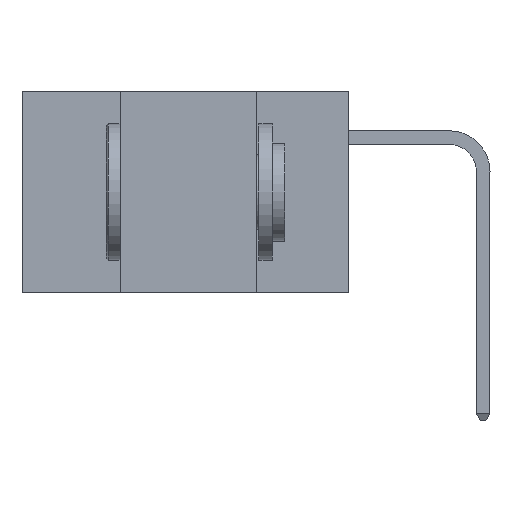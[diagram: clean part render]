
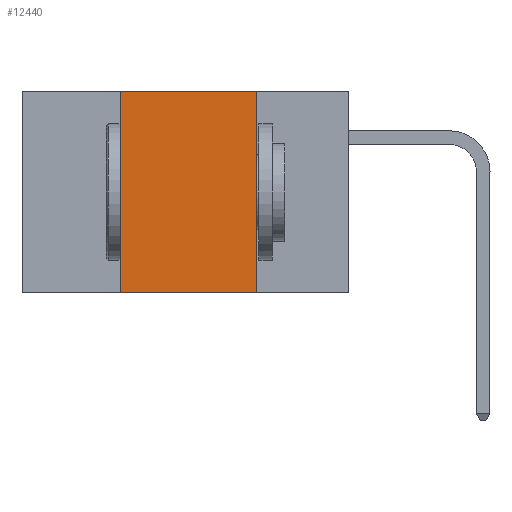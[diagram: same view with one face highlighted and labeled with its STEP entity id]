
A CAD part, left-side view. The second image highlights one B-rep face of the part: STEP entity #12440.
In plain terms, the highlighted planar face has unit normal (-1, 0, 0).
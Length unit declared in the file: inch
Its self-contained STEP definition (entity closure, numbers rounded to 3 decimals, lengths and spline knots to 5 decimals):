
#71 = CARTESIAN_POINT ( 'NONE',  ( 0., 0.6, 0. ) ) ;
#169 = DIRECTION ( 'NONE',  ( 1., 0., 0. ) ) ;
#422 = VECTOR ( 'NONE', #1328, 39.37008 ) ;
#915 = VERTEX_POINT ( 'NONE', #7883 ) ;
#1328 = DIRECTION ( 'NONE',  ( 0., 0., -1. ) ) ;
#1409 = CARTESIAN_POINT ( 'NONE',  ( 0., 0.17, 0. ) ) ;
#1415 = DIRECTION ( 'NONE',  ( 0., 0., 1. ) ) ;
#1425 = CARTESIAN_POINT ( 'NONE',  ( 0., 0.17, 0. ) ) ;
#1540 = EDGE_CURVE ( 'NONE', #2232, #915, #6671, .T. ) ;
#1567 = EDGE_CURVE ( 'NONE', #2153, #2232, #10754, .T. ) ;
#1773 = CARTESIAN_POINT ( 'NONE',  ( 0., 0.42, -0.37 ) ) ;
#2153 = VERTEX_POINT ( 'NONE', #8398 ) ;
#2232 = VERTEX_POINT ( 'NONE', #1425 ) ;
#4266 = VECTOR ( 'NONE', #1415, 39.37008 ) ;
#4402 = ORIENTED_EDGE ( 'NONE', *, *, #1540, .F. ) ;
#5175 = VECTOR ( 'NONE', #13646, 39.37008 ) ;
#5379 = DIRECTION ( 'NONE',  ( 0., 0., -1. ) ) ;
#5972 = LINE ( 'NONE', #6621, #5175 ) ;
#6589 = FACE_OUTER_BOUND ( 'NONE', #22274, .T. ) ;
#6621 = CARTESIAN_POINT ( 'NONE',  ( 0., 0.6, -0.37 ) ) ;
#6671 = LINE ( 'NONE', #1409, #422 ) ;
#6851 = ORIENTED_EDGE ( 'NONE', *, *, #19890, .T. ) ;
#7001 = CARTESIAN_POINT ( 'NONE',  ( 0., 0.6, 0. ) ) ;
#7883 = CARTESIAN_POINT ( 'NONE',  ( 0., 0.17, -0.37 ) ) ;
#8398 = CARTESIAN_POINT ( 'NONE',  ( 0., 0.42, 0. ) ) ;
#8587 = ORIENTED_EDGE ( 'NONE', *, *, #9890, .F. ) ;
#8912 = LINE ( 'NONE', #20785, #4266 ) ;
#9890 = EDGE_CURVE ( 'NONE', #21863, #2153, #8912, .T. ) ;
#10754 = LINE ( 'NONE', #71, #16823 ) ;
#11943 = DIRECTION ( 'NONE',  ( 0., -1., 0. ) ) ;
#12440 = ADVANCED_FACE ( 'NONE', ( #6589 ), #17500, .F. ) ;
#13646 = DIRECTION ( 'NONE',  ( 0., -1., 0. ) ) ;
#16823 = VECTOR ( 'NONE', #11943, 39.37008 ) ;
#17500 = PLANE ( 'NONE',  #21623 ) ;
#18060 = ORIENTED_EDGE ( 'NONE', *, *, #1567, .F. ) ;
#19890 = EDGE_CURVE ( 'NONE', #21863, #915, #5972, .T. ) ;
#20785 = CARTESIAN_POINT ( 'NONE',  ( 0., 0.42, 0. ) ) ;
#21623 = AXIS2_PLACEMENT_3D ( 'NONE', #7001, #169, #5379 ) ;
#21863 = VERTEX_POINT ( 'NONE', #1773 ) ;
#22274 = EDGE_LOOP ( 'NONE', ( #4402, #18060, #8587, #6851 ) ) ;
